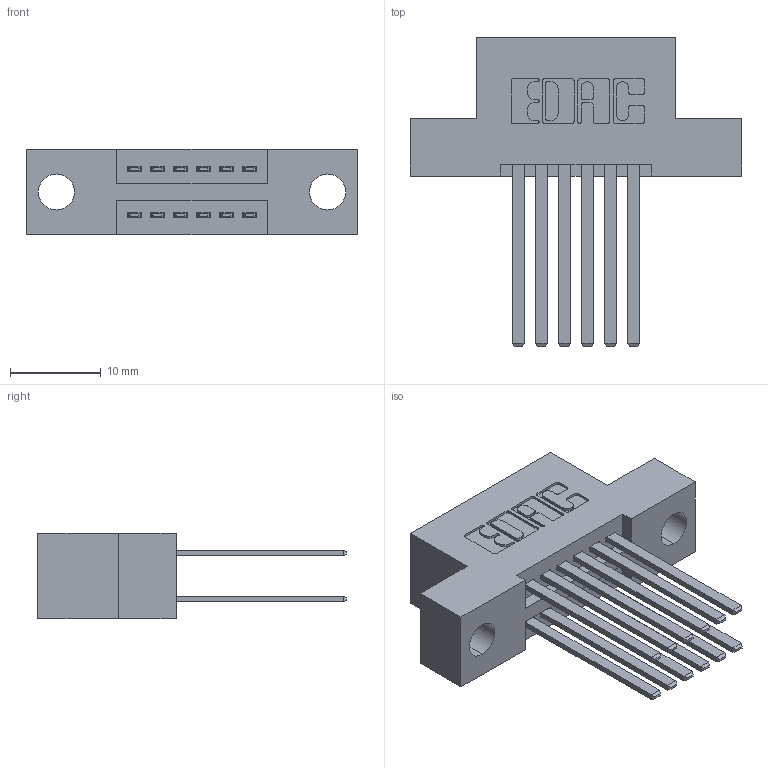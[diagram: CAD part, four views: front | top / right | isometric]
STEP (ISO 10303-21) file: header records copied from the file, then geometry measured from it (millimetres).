
FILE_DESCRIPTION (( 'STEP AP203' ), '1' );
FILE_NAME ('345-012-544-204.STEP', '2018-08-18T03:32:18', ( '' ), ( '' ), 'SwSTEP 2.0', 'SolidWorks 2016', '' );
FILE_SCHEMA (( 'CONFIG_CONTROL_DESIGN' ));
Length unit declared in the file: inch
Products named in the file (3): 345 Part_Flush Mounting Lugs - 0.156 Dia-TH; 345-292-001_345-293-144; 345-012-544-204
Assembly tree (13 placements, depth 2):
  345-012-544-204
    345 Part_Flush Mounting Lugs - 0.156 Dia-TH
    345-292-001_345-293-144  x12
Bounding box: 36.45 x 33.96 x 9.4 mm (x, y, z)
Volume: 3286.9 mm3; surface area: 4469.5 mm2
Topology: 13 solids, 13 shells, 654 faces, 1913 edges, 1258 vertices
Faces by surface type: plane 428, cylinder 226
Entity records: 9373 total; most frequent: CARTESIAN_POINT 1604, ORIENTED_EDGE 1538, DIRECTION 1457, EDGE_CURVE 769, VECTOR 617, LINE 617, VERTEX_POINT 510, AXIS2_PLACEMENT_3D 420
